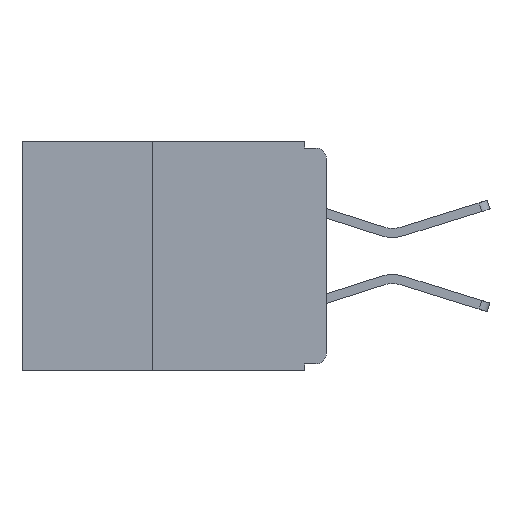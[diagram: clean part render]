
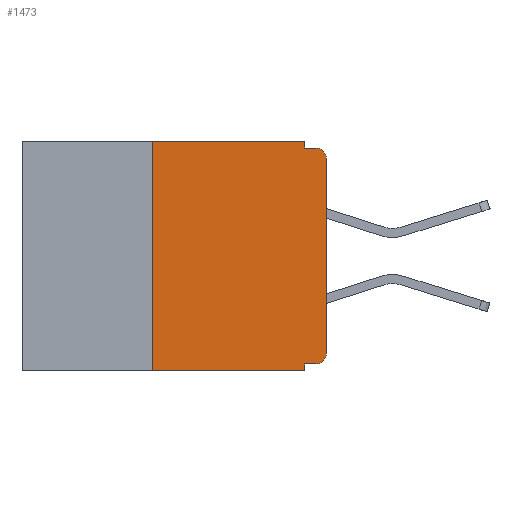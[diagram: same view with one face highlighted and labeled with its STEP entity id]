
A CAD part, left-side view. The second image highlights one B-rep face of the part: STEP entity #1473.
In plain terms, the highlighted planar face has unit normal (-1, 0, 0).
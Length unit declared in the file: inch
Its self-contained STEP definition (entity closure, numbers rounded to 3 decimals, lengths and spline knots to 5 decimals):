
#380 = ORIENTED_EDGE ( 'NONE', *, *, #22986, .T. ) ;
#850 = DIRECTION ( 'NONE',  ( 0., 0., 1. ) ) ;
#1021 = DIRECTION ( 'NONE',  ( 0., 0., -1. ) ) ;
#1048 = DIRECTION ( 'NONE',  ( -1., 0., 0. ) ) ;
#1075 = CARTESIAN_POINT ( 'NONE',  ( 0., 0.015, -0.025 ) ) ;
#1100 = ORIENTED_EDGE ( 'NONE', *, *, #8670, .F. ) ;
#1473 = ADVANCED_FACE ( 'NONE', ( #14421 ), #11363, .F. ) ;
#1521 = CARTESIAN_POINT ( 'NONE',  ( 0., 0.031, -0.01 ) ) ;
#2225 = VERTEX_POINT ( 'NONE', #21443 ) ;
#2373 = ORIENTED_EDGE ( 'NONE', *, *, #17417, .F. ) ;
#2429 = CARTESIAN_POINT ( 'NONE',  ( 0., 0.25, -0.33 ) ) ;
#2676 = EDGE_CURVE ( 'NONE', #4512, #5546, #23267, .T. ) ;
#2715 = LINE ( 'NONE', #20773, #7107 ) ;
#2993 = VECTOR ( 'NONE', #23097, 39.37008 ) ;
#3146 = ORIENTED_EDGE ( 'NONE', *, *, #9487, .F. ) ;
#3938 = CARTESIAN_POINT ( 'NONE',  ( 0., 0.437, 0. ) ) ;
#4172 = VECTOR ( 'NONE', #18848, 39.37008 ) ;
#4512 = VERTEX_POINT ( 'NONE', #15611 ) ;
#4698 = VERTEX_POINT ( 'NONE', #8423 ) ;
#4806 = CARTESIAN_POINT ( 'NONE',  ( 0., 0.437, -0.33 ) ) ;
#5546 = VERTEX_POINT ( 'NONE', #21631 ) ;
#5574 = LINE ( 'NONE', #6814, #14888 ) ;
#5743 = EDGE_CURVE ( 'NONE', #22889, #4698, #7580, .T. ) ;
#6095 = ORIENTED_EDGE ( 'NONE', *, *, #7639, .T. ) ;
#6132 = VERTEX_POINT ( 'NONE', #2429 ) ;
#6393 = ORIENTED_EDGE ( 'NONE', *, *, #2676, .F. ) ;
#6438 = DIRECTION ( 'NONE',  ( 0., -1., 0. ) ) ;
#6814 = CARTESIAN_POINT ( 'NONE',  ( 0., 0., -0.01 ) ) ;
#7107 = VECTOR ( 'NONE', #20503, 39.37008 ) ;
#7376 = AXIS2_PLACEMENT_3D ( 'NONE', #1075, #1048, #1021 ) ;
#7580 = LINE ( 'NONE', #14895, #21776 ) ;
#7639 = EDGE_CURVE ( 'NONE', #4512, #22292, #17073, .T. ) ;
#7962 = DIRECTION ( 'NONE',  ( 0., 0., -1. ) ) ;
#8011 = DIRECTION ( 'NONE',  ( -1., 0., 0. ) ) ;
#8036 = CARTESIAN_POINT ( 'NONE',  ( 0., 0.015, -0.305 ) ) ;
#8389 = CARTESIAN_POINT ( 'NONE',  ( 0., 0.25, -0.33 ) ) ;
#8423 = CARTESIAN_POINT ( 'NONE',  ( 0., 0.031, 0. ) ) ;
#8553 = CARTESIAN_POINT ( 'NONE',  ( 0., 0.031, -0.33 ) ) ;
#8620 = LINE ( 'NONE', #13513, #14102 ) ;
#8670 = EDGE_CURVE ( 'NONE', #5546, #10396, #8620, .T. ) ;
#9143 = LINE ( 'NONE', #19080, #4172 ) ;
#9366 = EDGE_CURVE ( 'NONE', #22292, #2225, #2715, .T. ) ;
#9487 = EDGE_CURVE ( 'NONE', #4698, #17677, #9143, .T. ) ;
#10360 = ORIENTED_EDGE ( 'NONE', *, *, #5743, .F. ) ;
#10396 = VERTEX_POINT ( 'NONE', #8553 ) ;
#10589 = EDGE_CURVE ( 'NONE', #17677, #23939, #5574, .T. ) ;
#11015 = EDGE_CURVE ( 'NONE', #2225, #23939, #20138, .T. ) ;
#11363 = PLANE ( 'NONE',  #11891 ) ;
#11891 = AXIS2_PLACEMENT_3D ( 'NONE', #3938, #12371, #12313 ) ;
#12313 = DIRECTION ( 'NONE',  ( 0., 0., -1. ) ) ;
#12371 = DIRECTION ( 'NONE',  ( 1., 0., 0. ) ) ;
#13409 = DIRECTION ( 'NONE',  ( 0., 0., -1. ) ) ;
#13513 = CARTESIAN_POINT ( 'NONE',  ( 0., 0.031, -0.33 ) ) ;
#14102 = VECTOR ( 'NONE', #13409, 39.37008 ) ;
#14313 = CARTESIAN_POINT ( 'NONE',  ( 0., 0.015, -0.01 ) ) ;
#14421 = FACE_OUTER_BOUND ( 'NONE', #17456, .T. ) ;
#14888 = VECTOR ( 'NONE', #6438, 39.37008 ) ;
#14895 = CARTESIAN_POINT ( 'NONE',  ( 0., 0.437, 0. ) ) ;
#14984 = DIRECTION ( 'NONE',  ( 0., -1., 0. ) ) ;
#15611 = CARTESIAN_POINT ( 'NONE',  ( 0., 0.015, -0.32 ) ) ;
#15625 = CARTESIAN_POINT ( 'NONE',  ( 0., 0.25, 0. ) ) ;
#15737 = CARTESIAN_POINT ( 'NONE',  ( 0., 0., -0.305 ) ) ;
#16061 = VECTOR ( 'NONE', #850, 39.37008 ) ;
#16414 = ORIENTED_EDGE ( 'NONE', *, *, #10589, .F. ) ;
#17073 = CIRCLE ( 'NONE', #21293, 0.015 ) ;
#17417 = EDGE_CURVE ( 'NONE', #6132, #22889, #20979, .T. ) ;
#17456 = EDGE_LOOP ( 'NONE', ( #18011, #17721, #16414, #3146, #10360, #2373, #380, #1100, #6393, #6095 ) ) ;
#17677 = VERTEX_POINT ( 'NONE', #1521 ) ;
#17721 = ORIENTED_EDGE ( 'NONE', *, *, #11015, .T. ) ;
#18011 = ORIENTED_EDGE ( 'NONE', *, *, #9366, .T. ) ;
#18689 = LINE ( 'NONE', #4806, #22971 ) ;
#18848 = DIRECTION ( 'NONE',  ( 0., 0., -1. ) ) ;
#19080 = CARTESIAN_POINT ( 'NONE',  ( 0., 0.031, 0. ) ) ;
#20138 = CIRCLE ( 'NONE', #7376, 0.015 ) ;
#20503 = DIRECTION ( 'NONE',  ( 0., 0., 1. ) ) ;
#20773 = CARTESIAN_POINT ( 'NONE',  ( 0., 0., 0. ) ) ;
#20979 = LINE ( 'NONE', #8389, #16061 ) ;
#21293 = AXIS2_PLACEMENT_3D ( 'NONE', #8036, #8011, #7962 ) ;
#21443 = CARTESIAN_POINT ( 'NONE',  ( 0., 0., -0.025 ) ) ;
#21532 = DIRECTION ( 'NONE',  ( 0., -1., 0. ) ) ;
#21631 = CARTESIAN_POINT ( 'NONE',  ( 0., 0.031, -0.32 ) ) ;
#21776 = VECTOR ( 'NONE', #14984, 39.37008 ) ;
#22292 = VERTEX_POINT ( 'NONE', #15737 ) ;
#22889 = VERTEX_POINT ( 'NONE', #15625 ) ;
#22971 = VECTOR ( 'NONE', #21532, 39.37008 ) ;
#22986 = EDGE_CURVE ( 'NONE', #6132, #10396, #18689, .T. ) ;
#22998 = CARTESIAN_POINT ( 'NONE',  ( 0., 0., -0.32 ) ) ;
#23097 = DIRECTION ( 'NONE',  ( 0., 1., 0. ) ) ;
#23267 = LINE ( 'NONE', #22998, #2993 ) ;
#23939 = VERTEX_POINT ( 'NONE', #14313 ) ;
